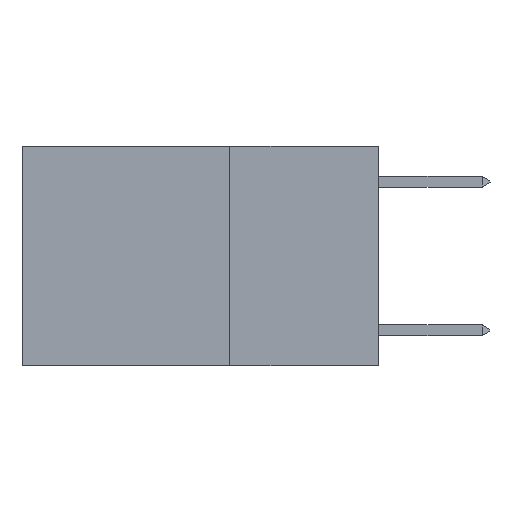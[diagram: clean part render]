
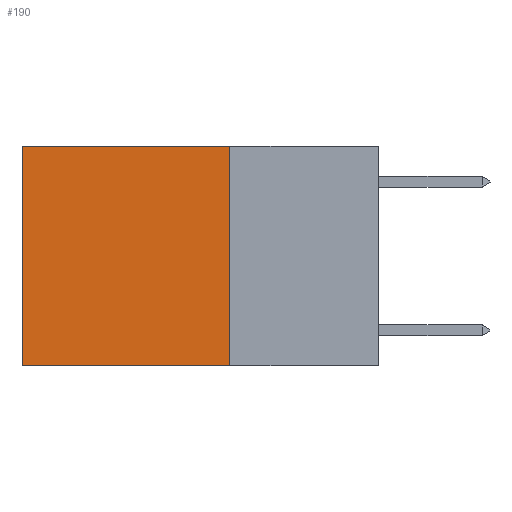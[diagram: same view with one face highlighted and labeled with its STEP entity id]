
A CAD part, left-side view. The second image highlights one B-rep face of the part: STEP entity #190.
In plain terms, the highlighted planar face has unit normal (-1, 0, 0).
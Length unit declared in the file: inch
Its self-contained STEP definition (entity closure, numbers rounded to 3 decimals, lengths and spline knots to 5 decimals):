
#190 = ADVANCED_FACE ( 'NONE', ( #15154 ), #11714, .F. ) ;
#2431 = LINE ( 'NONE', #16913, #6278 ) ;
#2590 = VECTOR ( 'NONE', #19642, 39.37008 ) ;
#2781 = AXIS2_PLACEMENT_3D ( 'NONE', #7029, #5961, #5890 ) ;
#2812 = VECTOR ( 'NONE', #15793, 39.37008 ) ;
#3044 = CARTESIAN_POINT ( 'NONE',  ( 0.2625, 0.25, -0.37 ) ) ;
#3837 = ORIENTED_EDGE ( 'NONE', *, *, #16666, .F. ) ;
#4605 = LINE ( 'NONE', #3044, #4847 ) ;
#4827 = EDGE_CURVE ( 'NONE', #15103, #18277, #4605, .T. ) ;
#4847 = VECTOR ( 'NONE', #16808, 39.37008 ) ;
#5408 = VERTEX_POINT ( 'NONE', #10695 ) ;
#5410 = CARTESIAN_POINT ( 'NONE',  ( 0.2625, 0.25, -0.37 ) ) ;
#5890 = DIRECTION ( 'NONE',  ( 0., 0., -1. ) ) ;
#5961 = DIRECTION ( 'NONE',  ( 1., 0., 0. ) ) ;
#6278 = VECTOR ( 'NONE', #7606, 39.37008 ) ;
#7029 = CARTESIAN_POINT ( 'NONE',  ( 0.2625, 0.25, 0. ) ) ;
#7606 = DIRECTION ( 'NONE',  ( 0., 0., -1. ) ) ;
#8614 = EDGE_CURVE ( 'NONE', #12127, #18277, #11686, .T. ) ;
#9556 = EDGE_CURVE ( 'NONE', #5408, #12127, #15487, .T. ) ;
#10230 = ORIENTED_EDGE ( 'NONE', *, *, #9556, .T. ) ;
#10695 = CARTESIAN_POINT ( 'NONE',  ( 0.2625, 0.25, 0. ) ) ;
#11686 = LINE ( 'NONE', #16633, #2590 ) ;
#11714 = PLANE ( 'NONE',  #2781 ) ;
#12127 = VERTEX_POINT ( 'NONE', #14107 ) ;
#12806 = CARTESIAN_POINT ( 'NONE',  ( 0.2625, 0.25, 0. ) ) ;
#12965 = ORIENTED_EDGE ( 'NONE', *, *, #4827, .F. ) ;
#13203 = CARTESIAN_POINT ( 'NONE',  ( 0.2625, 0.6, -0.37 ) ) ;
#14107 = CARTESIAN_POINT ( 'NONE',  ( 0.2625, 0.6, 0. ) ) ;
#14504 = ORIENTED_EDGE ( 'NONE', *, *, #8614, .T. ) ;
#15103 = VERTEX_POINT ( 'NONE', #5410 ) ;
#15154 = FACE_OUTER_BOUND ( 'NONE', #15592, .T. ) ;
#15487 = LINE ( 'NONE', #12806, #2812 ) ;
#15592 = EDGE_LOOP ( 'NONE', ( #14504, #12965, #3837, #10230 ) ) ;
#15793 = DIRECTION ( 'NONE',  ( 0., 1., 0. ) ) ;
#16633 = CARTESIAN_POINT ( 'NONE',  ( 0.2625, 0.6, 0. ) ) ;
#16666 = EDGE_CURVE ( 'NONE', #5408, #15103, #2431, .T. ) ;
#16808 = DIRECTION ( 'NONE',  ( 0., 1., 0. ) ) ;
#16913 = CARTESIAN_POINT ( 'NONE',  ( 0.2625, 0.25, 0. ) ) ;
#18277 = VERTEX_POINT ( 'NONE', #13203 ) ;
#19642 = DIRECTION ( 'NONE',  ( 0., 0., -1. ) ) ;
